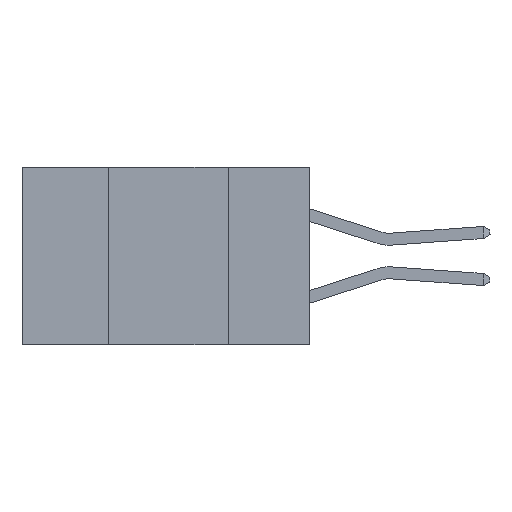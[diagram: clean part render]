
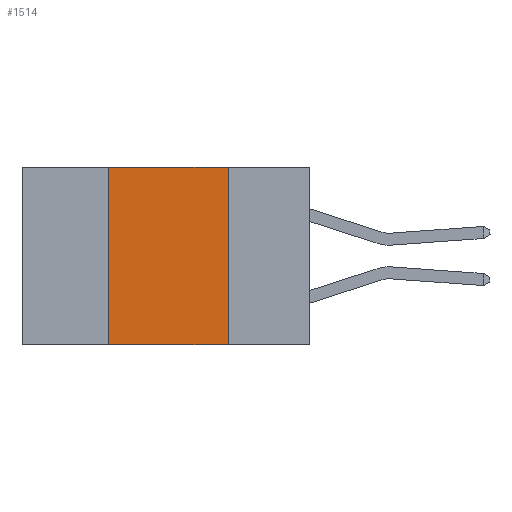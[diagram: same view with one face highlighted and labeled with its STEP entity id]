
A CAD part, left-side view. The second image highlights one B-rep face of the part: STEP entity #1514.
In plain terms, the highlighted planar face has unit normal (-1, 0, 0).
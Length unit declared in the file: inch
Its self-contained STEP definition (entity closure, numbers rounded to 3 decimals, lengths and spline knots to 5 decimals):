
#1514 = ADVANCED_FACE ( 'NONE', ( #25785 ), #27036, .F. ) ;
#2289 = LINE ( 'NONE', #21753, #27346 ) ;
#3241 = AXIS2_PLACEMENT_3D ( 'NONE', #11994, #19934, #19904 ) ;
#4125 = VERTEX_POINT ( 'NONE', #26077 ) ;
#4592 = VECTOR ( 'NONE', #30162, 39.37008 ) ;
#5154 = ORIENTED_EDGE ( 'NONE', *, *, #19068, .T. ) ;
#5703 = VERTEX_POINT ( 'NONE', #10158 ) ;
#7130 = EDGE_CURVE ( 'NONE', #14769, #17490, #2289, .T. ) ;
#7363 = DIRECTION ( 'NONE',  ( 0., 0., 1. ) ) ;
#8179 = CARTESIAN_POINT ( 'NONE',  ( 0., 0.17, 0. ) ) ;
#10158 = CARTESIAN_POINT ( 'NONE',  ( 0., 0.17, -0.37 ) ) ;
#11053 = LINE ( 'NONE', #17884, #24000 ) ;
#11994 = CARTESIAN_POINT ( 'NONE',  ( 0., 0.6, 0. ) ) ;
#12535 = DIRECTION ( 'NONE',  ( 0., -1., 0. ) ) ;
#14082 = VECTOR ( 'NONE', #20229, 39.37008 ) ;
#14601 = EDGE_CURVE ( 'NONE', #17490, #4125, #18226, .T. ) ;
#14769 = VERTEX_POINT ( 'NONE', #30673 ) ;
#14833 = LINE ( 'NONE', #8179, #14082 ) ;
#15743 = ORIENTED_EDGE ( 'NONE', *, *, #7130, .F. ) ;
#17490 = VERTEX_POINT ( 'NONE', #26834 ) ;
#17884 = CARTESIAN_POINT ( 'NONE',  ( 0., 0.6, -0.37 ) ) ;
#18226 = LINE ( 'NONE', #27770, #4592 ) ;
#18968 = EDGE_CURVE ( 'NONE', #4125, #5703, #14833, .T. ) ;
#19068 = EDGE_CURVE ( 'NONE', #14769, #5703, #11053, .T. ) ;
#19902 = ORIENTED_EDGE ( 'NONE', *, *, #14601, .F. ) ;
#19904 = DIRECTION ( 'NONE',  ( 0., 0., -1. ) ) ;
#19934 = DIRECTION ( 'NONE',  ( 1., 0., 0. ) ) ;
#20229 = DIRECTION ( 'NONE',  ( 0., 0., -1. ) ) ;
#21753 = CARTESIAN_POINT ( 'NONE',  ( 0., 0.42, 0. ) ) ;
#21780 = EDGE_LOOP ( 'NONE', ( #22570, #19902, #15743, #5154 ) ) ;
#22570 = ORIENTED_EDGE ( 'NONE', *, *, #18968, .F. ) ;
#24000 = VECTOR ( 'NONE', #12535, 39.37008 ) ;
#25785 = FACE_OUTER_BOUND ( 'NONE', #21780, .T. ) ;
#26077 = CARTESIAN_POINT ( 'NONE',  ( 0., 0.17, 0. ) ) ;
#26834 = CARTESIAN_POINT ( 'NONE',  ( 0., 0.42, 0. ) ) ;
#27036 = PLANE ( 'NONE',  #3241 ) ;
#27346 = VECTOR ( 'NONE', #7363, 39.37008 ) ;
#27770 = CARTESIAN_POINT ( 'NONE',  ( 0., 0.6, 0. ) ) ;
#30162 = DIRECTION ( 'NONE',  ( 0., -1., 0. ) ) ;
#30673 = CARTESIAN_POINT ( 'NONE',  ( 0., 0.42, -0.37 ) ) ;
